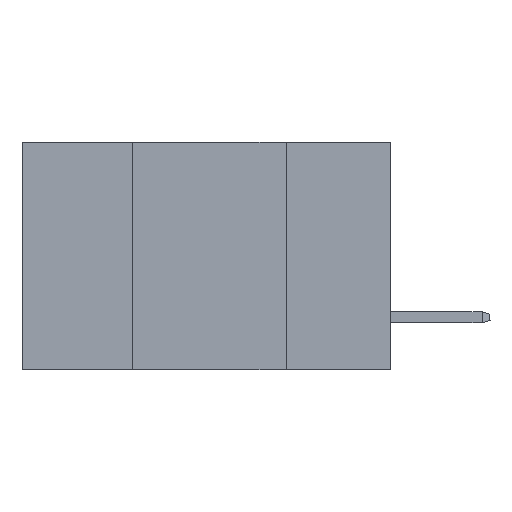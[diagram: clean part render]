
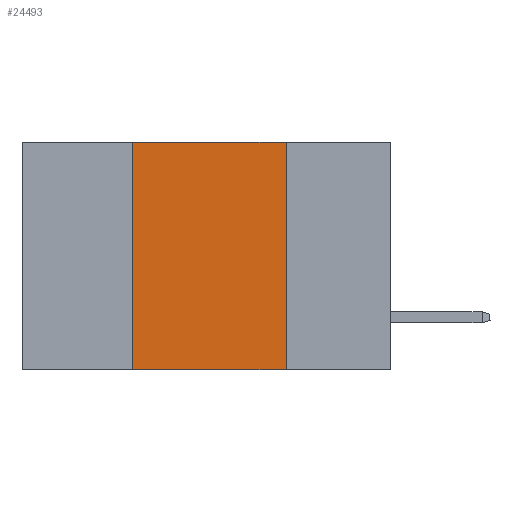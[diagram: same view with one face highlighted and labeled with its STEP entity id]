
A CAD part, left-side view. The second image highlights one B-rep face of the part: STEP entity #24493.
In plain terms, the highlighted planar face has unit normal (-1, 0, 0).
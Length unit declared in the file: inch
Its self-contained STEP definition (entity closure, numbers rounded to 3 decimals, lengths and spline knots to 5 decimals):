
#2143 = CARTESIAN_POINT ( 'NONE',  ( 0., 0.6, -0.37 ) ) ;
#2667 = CARTESIAN_POINT ( 'NONE',  ( 0., 0.42, -0.37 ) ) ;
#4609 = PLANE ( 'NONE',  #28694 ) ;
#5000 = CARTESIAN_POINT ( 'NONE',  ( 0., 0.17, 0. ) ) ;
#5002 = VERTEX_POINT ( 'NONE', #2667 ) ;
#5416 = ORIENTED_EDGE ( 'NONE', *, *, #22518, .F. ) ;
#5559 = ORIENTED_EDGE ( 'NONE', *, *, #26559, .F. ) ;
#6274 = VECTOR ( 'NONE', #8434, 39.37008 ) ;
#8402 = LINE ( 'NONE', #5000, #11723 ) ;
#8434 = DIRECTION ( 'NONE',  ( 0., 0., 1. ) ) ;
#10376 = LINE ( 'NONE', #2143, #18018 ) ;
#10694 = FACE_OUTER_BOUND ( 'NONE', #16595, .T. ) ;
#11613 = EDGE_CURVE ( 'NONE', #5002, #24735, #10376, .T. ) ;
#11723 = VECTOR ( 'NONE', #16625, 39.37008 ) ;
#11854 = EDGE_CURVE ( 'NONE', #30452, #24735, #8402, .T. ) ;
#13195 = DIRECTION ( 'NONE',  ( 0., 0., -1. ) ) ;
#13384 = DIRECTION ( 'NONE',  ( 1., 0., 0. ) ) ;
#15241 = ORIENTED_EDGE ( 'NONE', *, *, #11613, .T. ) ;
#16595 = EDGE_LOOP ( 'NONE', ( #26017, #5559, #5416, #15241 ) ) ;
#16625 = DIRECTION ( 'NONE',  ( 0., 0., -1. ) ) ;
#16998 = LINE ( 'NONE', #19856, #6274 ) ;
#17909 = DIRECTION ( 'NONE',  ( 0., -1., 0. ) ) ;
#18018 = VECTOR ( 'NONE', #17909, 39.37008 ) ;
#18709 = VERTEX_POINT ( 'NONE', #26656 ) ;
#18997 = DIRECTION ( 'NONE',  ( 0., -1., 0. ) ) ;
#19856 = CARTESIAN_POINT ( 'NONE',  ( 0., 0.42, 0. ) ) ;
#22518 = EDGE_CURVE ( 'NONE', #5002, #18709, #16998, .T. ) ;
#24493 = ADVANCED_FACE ( 'NONE', ( #10694 ), #4609, .F. ) ;
#24735 = VERTEX_POINT ( 'NONE', #32282 ) ;
#24740 = LINE ( 'NONE', #27590, #31075 ) ;
#26017 = ORIENTED_EDGE ( 'NONE', *, *, #11854, .F. ) ;
#26559 = EDGE_CURVE ( 'NONE', #18709, #30452, #24740, .T. ) ;
#26656 = CARTESIAN_POINT ( 'NONE',  ( 0., 0.42, 0. ) ) ;
#26976 = CARTESIAN_POINT ( 'NONE',  ( 0., 0.6, 0. ) ) ;
#27590 = CARTESIAN_POINT ( 'NONE',  ( 0., 0.6, 0. ) ) ;
#28694 = AXIS2_PLACEMENT_3D ( 'NONE', #26976, #13384, #13195 ) ;
#30452 = VERTEX_POINT ( 'NONE', #32078 ) ;
#31075 = VECTOR ( 'NONE', #18997, 39.37008 ) ;
#32078 = CARTESIAN_POINT ( 'NONE',  ( 0., 0.17, 0. ) ) ;
#32282 = CARTESIAN_POINT ( 'NONE',  ( 0., 0.17, -0.37 ) ) ;
